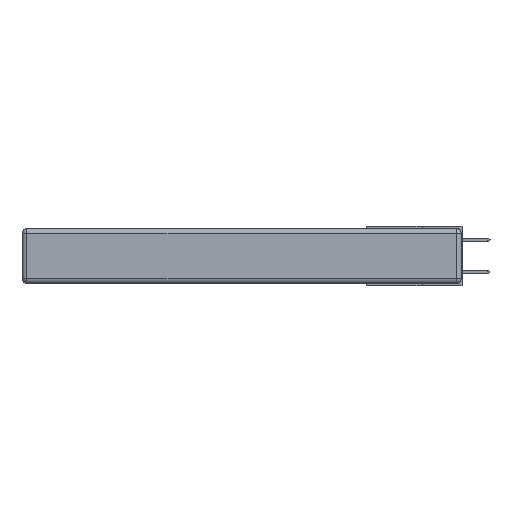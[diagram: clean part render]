
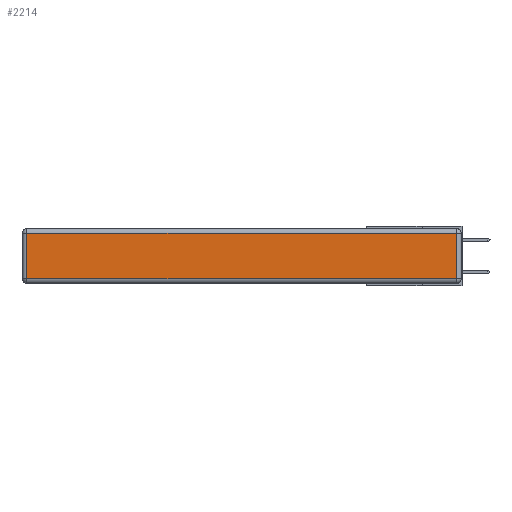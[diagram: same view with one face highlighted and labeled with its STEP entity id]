
A CAD part, left-side view. The second image highlights one B-rep face of the part: STEP entity #2214.
In plain terms, the highlighted planar face has unit normal (-1, 0, 0).
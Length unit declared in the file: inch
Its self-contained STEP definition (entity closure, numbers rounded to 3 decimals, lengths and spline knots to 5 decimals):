
#561 = DIRECTION ( 'NONE',  ( 0., 1., 0. ) ) ;
#576 = VERTEX_POINT ( 'NONE', #9936 ) ;
#1733 = LINE ( 'NONE', #28265, #18228 ) ;
#1866 = ORIENTED_EDGE ( 'NONE', *, *, #12404, .T. ) ;
#2214 = ADVANCED_FACE ( 'NONE', ( #19686 ), #26040, .T. ) ;
#2451 = VECTOR ( 'NONE', #22131, 39.37008 ) ;
#2517 = CARTESIAN_POINT ( 'NONE',  ( 0., 0., -0.313 ) ) ;
#3309 = AXIS2_PLACEMENT_3D ( 'NONE', #23689, #16476, #7435 ) ;
#3661 = ORIENTED_EDGE ( 'NONE', *, *, #13864, .T. ) ;
#3718 = CARTESIAN_POINT ( 'NONE',  ( 0., 2.72, -0.343 ) ) ;
#5104 = EDGE_CURVE ( 'NONE', #24037, #24594, #1733, .T. ) ;
#7086 = CARTESIAN_POINT ( 'NONE',  ( 0., 0.03, -0.343 ) ) ;
#7266 = EDGE_CURVE ( 'NONE', #576, #24037, #15923, .T. ) ;
#7321 = VECTOR ( 'NONE', #18825, 39.37008 ) ;
#7435 = DIRECTION ( 'NONE',  ( 0., 0., 1. ) ) ;
#9861 = EDGE_LOOP ( 'NONE', ( #1866, #12018, #15917, #3661 ) ) ;
#9936 = CARTESIAN_POINT ( 'NONE',  ( 0., 0.03, -0.313 ) ) ;
#10475 = LINE ( 'NONE', #3718, #2451 ) ;
#12018 = ORIENTED_EDGE ( 'NONE', *, *, #7266, .T. ) ;
#12404 = EDGE_CURVE ( 'NONE', #23558, #576, #13575, .T. ) ;
#12845 = CARTESIAN_POINT ( 'NONE',  ( 0., 0.03, -0.03 ) ) ;
#13575 = LINE ( 'NONE', #2517, #7321 ) ;
#13864 = EDGE_CURVE ( 'NONE', #24594, #23558, #10475, .T. ) ;
#15917 = ORIENTED_EDGE ( 'NONE', *, *, #5104, .T. ) ;
#15923 = LINE ( 'NONE', #7086, #25770 ) ;
#15937 = CARTESIAN_POINT ( 'NONE',  ( 0., 2.72, -0.03 ) ) ;
#16476 = DIRECTION ( 'NONE',  ( -1., 0., 0. ) ) ;
#18208 = CARTESIAN_POINT ( 'NONE',  ( 0., 2.72, -0.313 ) ) ;
#18228 = VECTOR ( 'NONE', #561, 39.37008 ) ;
#18825 = DIRECTION ( 'NONE',  ( 0., -1., 0. ) ) ;
#19686 = FACE_OUTER_BOUND ( 'NONE', #9861, .T. ) ;
#22131 = DIRECTION ( 'NONE',  ( 0., 0., -1. ) ) ;
#23558 = VERTEX_POINT ( 'NONE', #18208 ) ;
#23689 = CARTESIAN_POINT ( 'NONE',  ( 0., 0., -0.343 ) ) ;
#24037 = VERTEX_POINT ( 'NONE', #12845 ) ;
#24594 = VERTEX_POINT ( 'NONE', #15937 ) ;
#25770 = VECTOR ( 'NONE', #26381, 39.37008 ) ;
#26040 = PLANE ( 'NONE',  #3309 ) ;
#26381 = DIRECTION ( 'NONE',  ( 0., 0., 1. ) ) ;
#28265 = CARTESIAN_POINT ( 'NONE',  ( 0., 2.75, -0.03 ) ) ;
